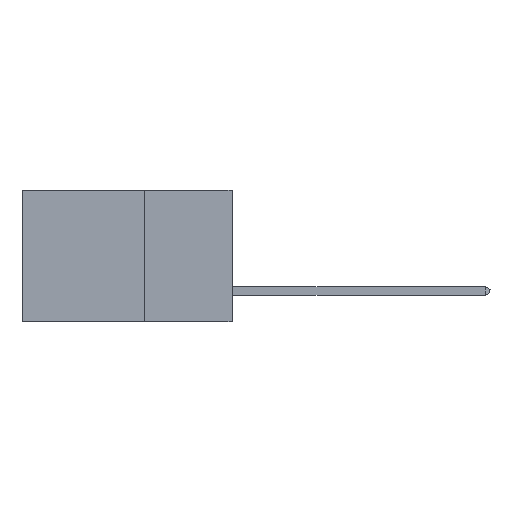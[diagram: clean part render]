
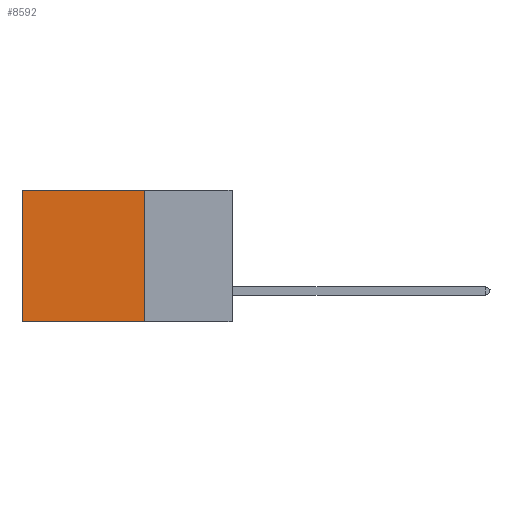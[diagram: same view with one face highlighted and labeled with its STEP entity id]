
A CAD part, left-side view. The second image highlights one B-rep face of the part: STEP entity #8592.
In plain terms, the highlighted planar face has unit normal (-1, 0, 0).
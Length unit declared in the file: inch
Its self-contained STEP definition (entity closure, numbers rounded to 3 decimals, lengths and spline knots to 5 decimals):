
#273 = EDGE_CURVE ( 'NONE', #11815, #16221, #10887, .T. ) ;
#366 = DIRECTION ( 'NONE',  ( 0., 0., -1. ) ) ;
#428 = FACE_OUTER_BOUND ( 'NONE', #9883, .T. ) ;
#484 = LINE ( 'NONE', #17876, #4593 ) ;
#1558 = VECTOR ( 'NONE', #6036, 39.37008 ) ;
#1766 = DIRECTION ( 'NONE',  ( 0., 1., 0. ) ) ;
#3169 = EDGE_CURVE ( 'NONE', #6409, #8358, #15275, .T. ) ;
#4420 = LINE ( 'NONE', #12693, #9894 ) ;
#4593 = VECTOR ( 'NONE', #1766, 39.37008 ) ;
#4613 = ORIENTED_EDGE ( 'NONE', *, *, #3169, .F. ) ;
#5693 = ORIENTED_EDGE ( 'NONE', *, *, #10807, .F. ) ;
#6036 = DIRECTION ( 'NONE',  ( 0., 0., -1. ) ) ;
#6184 = PLANE ( 'NONE',  #13809 ) ;
#6356 = VECTOR ( 'NONE', #10397, 39.37008 ) ;
#6409 = VERTEX_POINT ( 'NONE', #7964 ) ;
#6977 = CARTESIAN_POINT ( 'NONE',  ( 0.2875, 0.25, -0.375 ) ) ;
#7796 = CARTESIAN_POINT ( 'NONE',  ( 0.2875, 0.6, 0. ) ) ;
#7964 = CARTESIAN_POINT ( 'NONE',  ( 0.2875, 0.25, 0. ) ) ;
#8358 = VERTEX_POINT ( 'NONE', #6977 ) ;
#8592 = ADVANCED_FACE ( 'NONE', ( #428 ), #6184, .F. ) ;
#9883 = EDGE_LOOP ( 'NONE', ( #17926, #5693, #4613, #17684 ) ) ;
#9894 = VECTOR ( 'NONE', #11296, 39.37008 ) ;
#10397 = DIRECTION ( 'NONE',  ( 0., 0., -1. ) ) ;
#10807 = EDGE_CURVE ( 'NONE', #8358, #16221, #4420, .T. ) ;
#10887 = LINE ( 'NONE', #15662, #1558 ) ;
#11296 = DIRECTION ( 'NONE',  ( 0., 1., 0. ) ) ;
#11815 = VERTEX_POINT ( 'NONE', #7796 ) ;
#12693 = CARTESIAN_POINT ( 'NONE',  ( 0.2875, 0.25, -0.375 ) ) ;
#13074 = EDGE_CURVE ( 'NONE', #6409, #11815, #484, .T. ) ;
#13378 = CARTESIAN_POINT ( 'NONE',  ( 0.2875, 0.25, -0.375 ) ) ;
#13774 = CARTESIAN_POINT ( 'NONE',  ( 0.2875, 0.6, -0.375 ) ) ;
#13809 = AXIS2_PLACEMENT_3D ( 'NONE', #15802, #15926, #366 ) ;
#15275 = LINE ( 'NONE', #13378, #6356 ) ;
#15662 = CARTESIAN_POINT ( 'NONE',  ( 0.2875, 0.6, -0.375 ) ) ;
#15802 = CARTESIAN_POINT ( 'NONE',  ( 0.2875, 0.25, -0.375 ) ) ;
#15926 = DIRECTION ( 'NONE',  ( 1., 0., 0. ) ) ;
#16221 = VERTEX_POINT ( 'NONE', #13774 ) ;
#17684 = ORIENTED_EDGE ( 'NONE', *, *, #13074, .T. ) ;
#17876 = CARTESIAN_POINT ( 'NONE',  ( 0.2875, 0.25, 0. ) ) ;
#17926 = ORIENTED_EDGE ( 'NONE', *, *, #273, .T. ) ;
